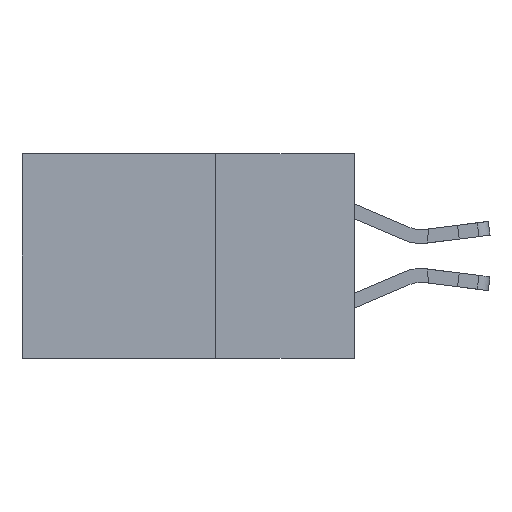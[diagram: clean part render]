
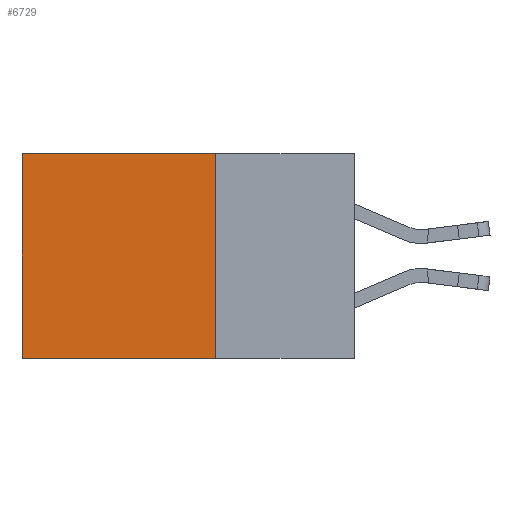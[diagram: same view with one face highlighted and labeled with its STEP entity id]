
A CAD part, left-side view. The second image highlights one B-rep face of the part: STEP entity #6729.
In plain terms, the highlighted planar face has unit normal (-1, 0, 0).
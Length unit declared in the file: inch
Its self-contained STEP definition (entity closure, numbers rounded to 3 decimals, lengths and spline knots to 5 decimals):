
#403 = VECTOR ( 'NONE', #4339, 39.37008 ) ;
#1704 = AXIS2_PLACEMENT_3D ( 'NONE', #6192, #11665, #11821 ) ;
#2427 = CARTESIAN_POINT ( 'NONE',  ( 0.298, 0.25, -0.37 ) ) ;
#2817 = CARTESIAN_POINT ( 'NONE',  ( 0.298, 0.25, 0. ) ) ;
#2867 = LINE ( 'NONE', #2817, #19071 ) ;
#3601 = VERTEX_POINT ( 'NONE', #9386 ) ;
#4339 = DIRECTION ( 'NONE',  ( 0., 1., 0. ) ) ;
#4398 = CARTESIAN_POINT ( 'NONE',  ( 0.298, 0.25, 0. ) ) ;
#5213 = ORIENTED_EDGE ( 'NONE', *, *, #14882, .T. ) ;
#5316 = VECTOR ( 'NONE', #6389, 39.37008 ) ;
#6192 = CARTESIAN_POINT ( 'NONE',  ( 0.298, 0.25, 0. ) ) ;
#6389 = DIRECTION ( 'NONE',  ( 0., 1., 0. ) ) ;
#6729 = ADVANCED_FACE ( 'NONE', ( #15121 ), #9726, .F. ) ;
#6855 = LINE ( 'NONE', #2427, #403 ) ;
#6991 = VERTEX_POINT ( 'NONE', #10768 ) ;
#7076 = ORIENTED_EDGE ( 'NONE', *, *, #18218, .T. ) ;
#9386 = CARTESIAN_POINT ( 'NONE',  ( 0.298, 0.6, -0.37 ) ) ;
#9726 = PLANE ( 'NONE',  #1704 ) ;
#10022 = CARTESIAN_POINT ( 'NONE',  ( 0.298, 0.6, 0. ) ) ;
#10692 = EDGE_LOOP ( 'NONE', ( #5213, #18654, #18422, #7076 ) ) ;
#10768 = CARTESIAN_POINT ( 'NONE',  ( 0.298, 0.6, 0. ) ) ;
#11665 = DIRECTION ( 'NONE',  ( 1., 0., 0. ) ) ;
#11821 = DIRECTION ( 'NONE',  ( 0., 0., -1. ) ) ;
#12668 = CARTESIAN_POINT ( 'NONE',  ( 0.298, 0.25, -0.37 ) ) ;
#14374 = VERTEX_POINT ( 'NONE', #18536 ) ;
#14882 = EDGE_CURVE ( 'NONE', #6991, #3601, #15825, .T. ) ;
#15121 = FACE_OUTER_BOUND ( 'NONE', #10692, .T. ) ;
#15825 = LINE ( 'NONE', #10022, #18071 ) ;
#18071 = VECTOR ( 'NONE', #20623, 39.37008 ) ;
#18218 = EDGE_CURVE ( 'NONE', #14374, #6991, #19602, .T. ) ;
#18422 = ORIENTED_EDGE ( 'NONE', *, *, #23041, .F. ) ;
#18536 = CARTESIAN_POINT ( 'NONE',  ( 0.298, 0.25, 0. ) ) ;
#18654 = ORIENTED_EDGE ( 'NONE', *, *, #22116, .F. ) ;
#18984 = DIRECTION ( 'NONE',  ( 0., 0., -1. ) ) ;
#19071 = VECTOR ( 'NONE', #18984, 39.37008 ) ;
#19222 = VERTEX_POINT ( 'NONE', #12668 ) ;
#19602 = LINE ( 'NONE', #4398, #5316 ) ;
#20623 = DIRECTION ( 'NONE',  ( 0., 0., -1. ) ) ;
#22116 = EDGE_CURVE ( 'NONE', #19222, #3601, #6855, .T. ) ;
#23041 = EDGE_CURVE ( 'NONE', #14374, #19222, #2867, .T. ) ;
